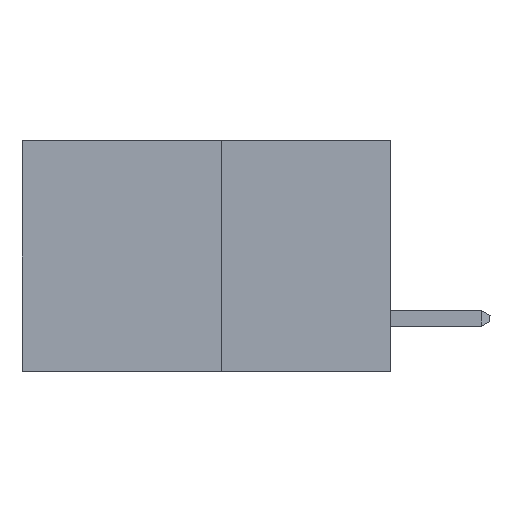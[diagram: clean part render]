
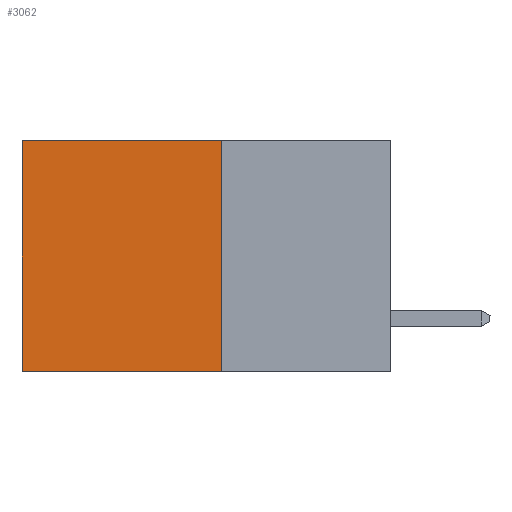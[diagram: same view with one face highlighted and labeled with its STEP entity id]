
A CAD part, left-side view. The second image highlights one B-rep face of the part: STEP entity #3062.
In plain terms, the highlighted planar face has unit normal (-1, 0, 0).
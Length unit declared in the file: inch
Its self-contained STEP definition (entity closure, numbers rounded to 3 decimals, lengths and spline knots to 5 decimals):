
#482 = CARTESIAN_POINT ( 'NONE',  ( 0.277, 0.59, 0. ) ) ;
#787 = VECTOR ( 'NONE', #4182, 39.37008 ) ;
#854 = VERTEX_POINT ( 'NONE', #482 ) ;
#1014 = DIRECTION ( 'NONE',  ( 1., 0., 0. ) ) ;
#1716 = VERTEX_POINT ( 'NONE', #6516 ) ;
#2018 = CARTESIAN_POINT ( 'NONE',  ( 0.277, 0.27, -0.37 ) ) ;
#2270 = ORIENTED_EDGE ( 'NONE', *, *, #5770, .T. ) ;
#3062 = ADVANCED_FACE ( 'NONE', ( #6090 ), #4919, .F. ) ;
#3223 = EDGE_LOOP ( 'NONE', ( #2270, #7444, #5396, #4818 ) ) ;
#3325 = CARTESIAN_POINT ( 'NONE',  ( 0.277, 0.59, -0.37 ) ) ;
#3496 = VERTEX_POINT ( 'NONE', #8256 ) ;
#3998 = CARTESIAN_POINT ( 'NONE',  ( 0.277, 0.59, -0.37 ) ) ;
#4182 = DIRECTION ( 'NONE',  ( 0., 0., -1. ) ) ;
#4728 = DIRECTION ( 'NONE',  ( 0., 1., 0. ) ) ;
#4774 = EDGE_CURVE ( 'NONE', #3496, #854, #9217, .T. ) ;
#4802 = LINE ( 'NONE', #2018, #6936 ) ;
#4818 = ORIENTED_EDGE ( 'NONE', *, *, #4774, .T. ) ;
#4919 = PLANE ( 'NONE',  #8995 ) ;
#4967 = EDGE_CURVE ( 'NONE', #3496, #1716, #4802, .T. ) ;
#5287 = LINE ( 'NONE', #3325, #787 ) ;
#5396 = ORIENTED_EDGE ( 'NONE', *, *, #4967, .F. ) ;
#5770 = EDGE_CURVE ( 'NONE', #854, #7547, #5287, .T. ) ;
#6090 = FACE_OUTER_BOUND ( 'NONE', #3223, .T. ) ;
#6516 = CARTESIAN_POINT ( 'NONE',  ( 0.277, 0.27, -0.37 ) ) ;
#6815 = VECTOR ( 'NONE', #10049, 39.37008 ) ;
#6936 = VECTOR ( 'NONE', #7785, 39.37008 ) ;
#7258 = LINE ( 'NONE', #7923, #9173 ) ;
#7442 = EDGE_CURVE ( 'NONE', #1716, #7547, #7258, .T. ) ;
#7444 = ORIENTED_EDGE ( 'NONE', *, *, #7442, .F. ) ;
#7547 = VERTEX_POINT ( 'NONE', #3998 ) ;
#7785 = DIRECTION ( 'NONE',  ( 0., 0., -1. ) ) ;
#7923 = CARTESIAN_POINT ( 'NONE',  ( 0.277, 0.27, -0.37 ) ) ;
#8094 = CARTESIAN_POINT ( 'NONE',  ( 0.277, 0.27, -0.37 ) ) ;
#8179 = DIRECTION ( 'NONE',  ( 0., 0., -1. ) ) ;
#8256 = CARTESIAN_POINT ( 'NONE',  ( 0.277, 0.27, 0. ) ) ;
#8995 = AXIS2_PLACEMENT_3D ( 'NONE', #8094, #1014, #8179 ) ;
#9173 = VECTOR ( 'NONE', #4728, 39.37008 ) ;
#9217 = LINE ( 'NONE', #9873, #6815 ) ;
#9873 = CARTESIAN_POINT ( 'NONE',  ( 0.277, 0.27, 0. ) ) ;
#10049 = DIRECTION ( 'NONE',  ( 0., 1., 0. ) ) ;
